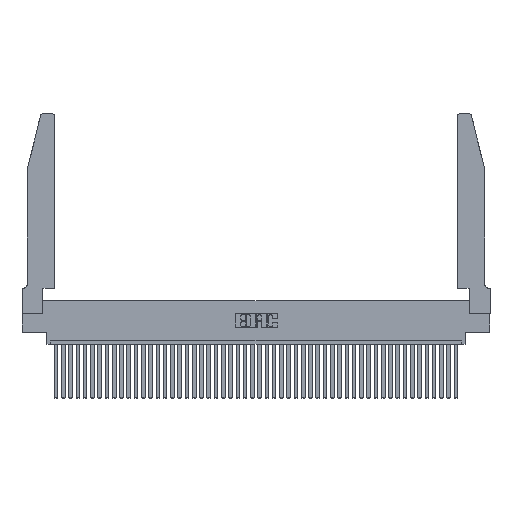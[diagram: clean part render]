
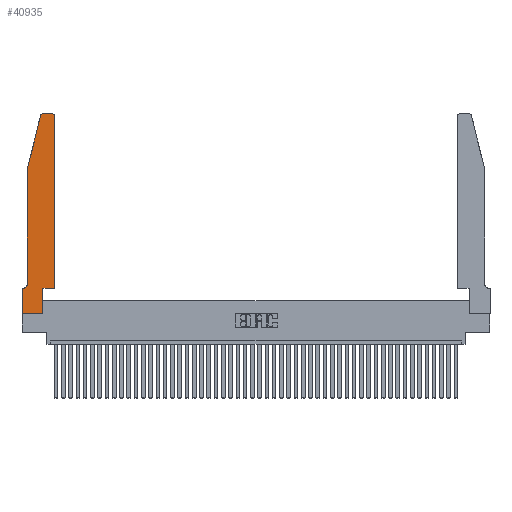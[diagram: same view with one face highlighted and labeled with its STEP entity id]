
A CAD part, top view. The second image highlights one B-rep face of the part: STEP entity #40935.
In plain terms, the highlighted planar face has unit normal (0, 0, 1).
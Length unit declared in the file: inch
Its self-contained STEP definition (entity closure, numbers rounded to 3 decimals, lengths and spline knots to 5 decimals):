
#637 = VERTEX_POINT ( 'NONE', #22116 ) ;
#740 = DIRECTION ( 'NONE',  ( 0., -1., 0. ) ) ;
#1872 = CARTESIAN_POINT ( 'NONE',  ( 0.4205, 2.72, 0.37 ) ) ;
#2347 = VERTEX_POINT ( 'NONE', #27897 ) ;
#3277 = VECTOR ( 'NONE', #11121, 39.37008 ) ;
#3684 = EDGE_CURVE ( 'NONE', #24975, #32942, #33610, .T. ) ;
#3874 = LINE ( 'NONE', #38499, #8263 ) ;
#4209 = CARTESIAN_POINT ( 'NONE',  ( 0.0755, 2., 0.37 ) ) ;
#4368 = CARTESIAN_POINT ( 'NONE',  ( 0.0755, 2., 0.37 ) ) ;
#4413 = VERTEX_POINT ( 'NONE', #16494 ) ;
#4632 = DIRECTION ( 'NONE',  ( 0., 0., 1. ) ) ;
#4729 = CARTESIAN_POINT ( 'NONE',  ( 0., 0., 0.37 ) ) ;
#4754 = LINE ( 'NONE', #35431, #25881 ) ;
#5271 = ORIENTED_EDGE ( 'NONE', *, *, #13119, .T. ) ;
#5910 = ORIENTED_EDGE ( 'NONE', *, *, #30682, .T. ) ;
#6592 = ORIENTED_EDGE ( 'NONE', *, *, #29839, .T. ) ;
#6924 = DIRECTION ( 'NONE',  ( -1., 0., 0. ) ) ;
#8263 = VECTOR ( 'NONE', #41705, 39.37008 ) ;
#8838 = LINE ( 'NONE', #33421, #27754 ) ;
#10708 = VECTOR ( 'NONE', #31620, 39.37008 ) ;
#10884 = VERTEX_POINT ( 'NONE', #31589 ) ;
#11121 = DIRECTION ( 'NONE',  ( 1., 0., 0. ) ) ;
#11396 = DIRECTION ( 'NONE',  ( 0., -1., 0. ) ) ;
#12769 = VERTEX_POINT ( 'NONE', #22700 ) ;
#13119 = EDGE_CURVE ( 'NONE', #10884, #4413, #20648, .T. ) ;
#14341 = CARTESIAN_POINT ( 'NONE',  ( 0.4505, 0.35, 0.37 ) ) ;
#14627 = ORIENTED_EDGE ( 'NONE', *, *, #31304, .T. ) ;
#15051 = EDGE_CURVE ( 'NONE', #4413, #2347, #15557, .T. ) ;
#15316 = AXIS2_PLACEMENT_3D ( 'NONE', #37937, #41435, #6924 ) ;
#15557 = LINE ( 'NONE', #40425, #42051 ) ;
#16452 = DIRECTION ( 'NONE',  ( 1., 0., 0. ) ) ;
#16494 = CARTESIAN_POINT ( 'NONE',  ( 0.4205, 2.75, 0.37 ) ) ;
#17237 = ORIENTED_EDGE ( 'NONE', *, *, #20158, .T. ) ;
#18279 = FACE_OUTER_BOUND ( 'NONE', #35163, .T. ) ;
#19301 = LINE ( 'NONE', #4368, #39269 ) ;
#19319 = VERTEX_POINT ( 'NONE', #24472 ) ;
#19903 = LINE ( 'NONE', #31684, #39355 ) ;
#20158 = EDGE_CURVE ( 'NONE', #12769, #37164, #4754, .T. ) ;
#20338 = CARTESIAN_POINT ( 'NONE',  ( 0.0055, 0.35, 0.37 ) ) ;
#20526 = CARTESIAN_POINT ( 'NONE',  ( 0.2865, 0., 0.37 ) ) ;
#20648 = CIRCLE ( 'NONE', #26013, 0.03 ) ;
#21739 = ORIENTED_EDGE ( 'NONE', *, *, #15051, .T. ) ;
#22116 = CARTESIAN_POINT ( 'NONE',  ( 0.25487, 2.72718, 0.37 ) ) ;
#22445 = CARTESIAN_POINT ( 'NONE',  ( 0.2865, 0.35, 0.37 ) ) ;
#22689 = DIRECTION ( 'NONE',  ( -1., 0., 0. ) ) ;
#22700 = CARTESIAN_POINT ( 'NONE',  ( 0., 0.35, 0.37 ) ) ;
#23048 = CIRCLE ( 'NONE', #15316, 0.07 ) ;
#23517 = ORIENTED_EDGE ( 'NONE', *, *, #42045, .T. ) ;
#24472 = CARTESIAN_POINT ( 'NONE',  ( 0.0755, 0.42, 0.37 ) ) ;
#24884 = AXIS2_PLACEMENT_3D ( 'NONE', #41500, #34371, #37862 ) ;
#24975 = VERTEX_POINT ( 'NONE', #22445 ) ;
#25552 = EDGE_CURVE ( 'NONE', #637, #27935, #32349, .T. ) ;
#25689 = ORIENTED_EDGE ( 'NONE', *, *, #25552, .T. ) ;
#25825 = ORIENTED_EDGE ( 'NONE', *, *, #43346, .T. ) ;
#25881 = VECTOR ( 'NONE', #740, 39.37008 ) ;
#26013 = AXIS2_PLACEMENT_3D ( 'NONE', #1872, #4632, #28848 ) ;
#26473 = VERTEX_POINT ( 'NONE', #20526 ) ;
#27255 = EDGE_CURVE ( 'NONE', #2347, #637, #28214, .T. ) ;
#27281 = VECTOR ( 'NONE', #31231, 39.37008 ) ;
#27754 = VECTOR ( 'NONE', #22689, 39.37008 ) ;
#27897 = CARTESIAN_POINT ( 'NONE',  ( 0.284, 2.75, 0.37 ) ) ;
#27935 = VERTEX_POINT ( 'NONE', #41591 ) ;
#28214 = CIRCLE ( 'NONE', #24884, 0.03 ) ;
#28848 = DIRECTION ( 'NONE',  ( 1., 0., 0. ) ) ;
#29691 = PLANE ( 'NONE',  #44263 ) ;
#29839 = EDGE_CURVE ( 'NONE', #26473, #24975, #19903, .T. ) ;
#30682 = EDGE_CURVE ( 'NONE', #27935, #19319, #19301, .T. ) ;
#31231 = DIRECTION ( 'NONE',  ( 1., 0., 0. ) ) ;
#31304 = EDGE_CURVE ( 'NONE', #37164, #26473, #34896, .T. ) ;
#31589 = CARTESIAN_POINT ( 'NONE',  ( 0.4505, 2.72, 0.37 ) ) ;
#31620 = DIRECTION ( 'NONE',  ( -0.239, -0.971, 0. ) ) ;
#31684 = CARTESIAN_POINT ( 'NONE',  ( 0.2865, 0.35, 0.37 ) ) ;
#32349 = LINE ( 'NONE', #4209, #10708 ) ;
#32942 = VERTEX_POINT ( 'NONE', #43844 ) ;
#33342 = DIRECTION ( 'NONE',  ( 0., 0., 1. ) ) ;
#33421 = CARTESIAN_POINT ( 'NONE',  ( 0.0755, 0.35, 0.37 ) ) ;
#33610 = LINE ( 'NONE', #14341, #3277 ) ;
#34371 = DIRECTION ( 'NONE',  ( 0., 0., 1. ) ) ;
#34500 = ORIENTED_EDGE ( 'NONE', *, *, #3684, .T. ) ;
#34896 = LINE ( 'NONE', #4729, #27281 ) ;
#35163 = EDGE_LOOP ( 'NONE', ( #21739, #43332, #25689, #5910, #23517, #25825, #17237, #14627, #6592, #34500, #37078, #5271 ) ) ;
#35365 = VERTEX_POINT ( 'NONE', #20338 ) ;
#35431 = CARTESIAN_POINT ( 'NONE',  ( 0., 0., 0.37 ) ) ;
#36548 = EDGE_CURVE ( 'NONE', #32942, #10884, #3874, .T. ) ;
#36670 = CARTESIAN_POINT ( 'NONE',  ( 0., 0.35, 0.37 ) ) ;
#37078 = ORIENTED_EDGE ( 'NONE', *, *, #36548, .T. ) ;
#37164 = VERTEX_POINT ( 'NONE', #38404 ) ;
#37862 = DIRECTION ( 'NONE',  ( 1., 0., 0. ) ) ;
#37937 = CARTESIAN_POINT ( 'NONE',  ( 0.0055, 0.42, 0.37 ) ) ;
#38200 = DIRECTION ( 'NONE',  ( 0., 1., 0. ) ) ;
#38404 = CARTESIAN_POINT ( 'NONE',  ( 0., 0., 0.37 ) ) ;
#38499 = CARTESIAN_POINT ( 'NONE',  ( 0.4505, 0.35, 0.37 ) ) ;
#39269 = VECTOR ( 'NONE', #11396, 39.37008 ) ;
#39355 = VECTOR ( 'NONE', #38200, 39.37008 ) ;
#40135 = DIRECTION ( 'NONE',  ( -1., 0., 0. ) ) ;
#40425 = CARTESIAN_POINT ( 'NONE',  ( 0.2605, 2.75, 0.37 ) ) ;
#40935 = ADVANCED_FACE ( 'NONE', ( #18279 ), #29691, .T. ) ;
#41435 = DIRECTION ( 'NONE',  ( 0., 0., -1. ) ) ;
#41500 = CARTESIAN_POINT ( 'NONE',  ( 0.284, 2.72, 0.37 ) ) ;
#41591 = CARTESIAN_POINT ( 'NONE',  ( 0.0755, 2., 0.37 ) ) ;
#41705 = DIRECTION ( 'NONE',  ( 0., 1., 0. ) ) ;
#42045 = EDGE_CURVE ( 'NONE', #19319, #35365, #23048, .T. ) ;
#42051 = VECTOR ( 'NONE', #40135, 39.37008 ) ;
#43332 = ORIENTED_EDGE ( 'NONE', *, *, #27255, .T. ) ;
#43346 = EDGE_CURVE ( 'NONE', #35365, #12769, #8838, .T. ) ;
#43844 = CARTESIAN_POINT ( 'NONE',  ( 0.4505, 0.35, 0.37 ) ) ;
#44263 = AXIS2_PLACEMENT_3D ( 'NONE', #36670, #33342, #16452 ) ;
